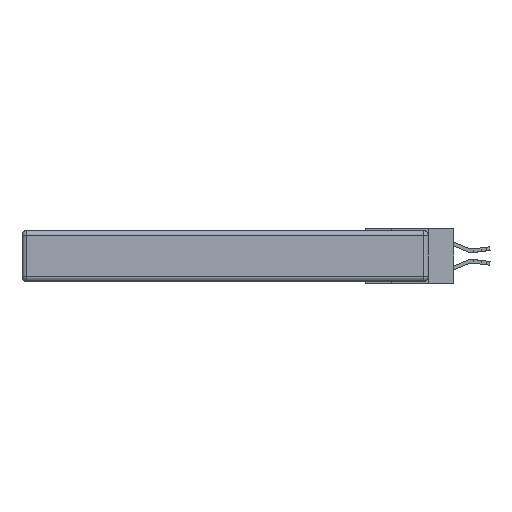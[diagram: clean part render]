
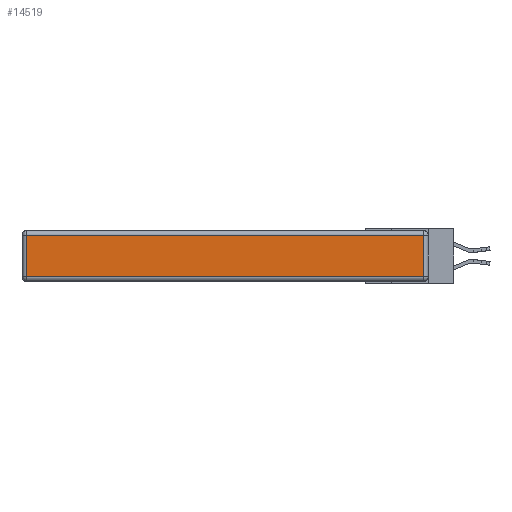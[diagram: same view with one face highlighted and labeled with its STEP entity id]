
A CAD part, left-side view. The second image highlights one B-rep face of the part: STEP entity #14519.
In plain terms, the highlighted planar face has unit normal (-1, 0, 0).
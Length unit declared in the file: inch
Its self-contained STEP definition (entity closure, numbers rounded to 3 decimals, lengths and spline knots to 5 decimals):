
#67 = VERTEX_POINT ( 'NONE', #11127 ) ;
#92 = CARTESIAN_POINT ( 'NONE',  ( 0., 0.03, -0.313 ) ) ;
#482 = LINE ( 'NONE', #483, #11576 ) ;
#483 = CARTESIAN_POINT ( 'NONE',  ( 0., 0.03, -0.343 ) ) ;
#644 = DIRECTION ( 'NONE',  ( 0., 1., 0. ) ) ;
#2622 = ORIENTED_EDGE ( 'NONE', *, *, #9029, .T. ) ;
#2682 = AXIS2_PLACEMENT_3D ( 'NONE', #15632, #15689, #5645 ) ;
#3891 = EDGE_CURVE ( 'NONE', #11173, #67, #482, .T. ) ;
#4084 = ORIENTED_EDGE ( 'NONE', *, *, #3891, .T. ) ;
#4220 = ORIENTED_EDGE ( 'NONE', *, *, #16391, .T. ) ;
#5066 = LINE ( 'NONE', #6367, #6274 ) ;
#5645 = DIRECTION ( 'NONE',  ( 0., 0., 1. ) ) ;
#6274 = VECTOR ( 'NONE', #7625, 39.37008 ) ;
#6367 = CARTESIAN_POINT ( 'NONE',  ( 0., 0., -0.313 ) ) ;
#6748 = PLANE ( 'NONE',  #2682 ) ;
#7036 = DIRECTION ( 'NONE',  ( 0., 0., -1. ) ) ;
#7625 = DIRECTION ( 'NONE',  ( 0., -1., 0. ) ) ;
#9029 = EDGE_CURVE ( 'NONE', #67, #14883, #10193, .T. ) ;
#9389 = VERTEX_POINT ( 'NONE', #14616 ) ;
#10193 = LINE ( 'NONE', #13376, #14774 ) ;
#10432 = EDGE_LOOP ( 'NONE', ( #4220, #4084, #2622, #14399 ) ) ;
#11127 = CARTESIAN_POINT ( 'NONE',  ( 0., 0.03, -0.03 ) ) ;
#11173 = VERTEX_POINT ( 'NONE', #92 ) ;
#11193 = LINE ( 'NONE', #14629, #13573 ) ;
#11214 = FACE_OUTER_BOUND ( 'NONE', #10432, .T. ) ;
#11576 = VECTOR ( 'NONE', #15717, 39.37008 ) ;
#12957 = CARTESIAN_POINT ( 'NONE',  ( 0., 2.72, -0.03 ) ) ;
#13376 = CARTESIAN_POINT ( 'NONE',  ( 0., 2.75, -0.03 ) ) ;
#13573 = VECTOR ( 'NONE', #7036, 39.37008 ) ;
#14399 = ORIENTED_EDGE ( 'NONE', *, *, #14651, .T. ) ;
#14519 = ADVANCED_FACE ( 'NONE', ( #11214 ), #6748, .T. ) ;
#14616 = CARTESIAN_POINT ( 'NONE',  ( 0., 2.72, -0.313 ) ) ;
#14629 = CARTESIAN_POINT ( 'NONE',  ( 0., 2.72, -0.343 ) ) ;
#14651 = EDGE_CURVE ( 'NONE', #14883, #9389, #11193, .T. ) ;
#14774 = VECTOR ( 'NONE', #644, 39.37008 ) ;
#14883 = VERTEX_POINT ( 'NONE', #12957 ) ;
#15632 = CARTESIAN_POINT ( 'NONE',  ( 0., 0., -0.343 ) ) ;
#15689 = DIRECTION ( 'NONE',  ( -1., 0., 0. ) ) ;
#15717 = DIRECTION ( 'NONE',  ( 0., 0., 1. ) ) ;
#16391 = EDGE_CURVE ( 'NONE', #9389, #11173, #5066, .T. ) ;
